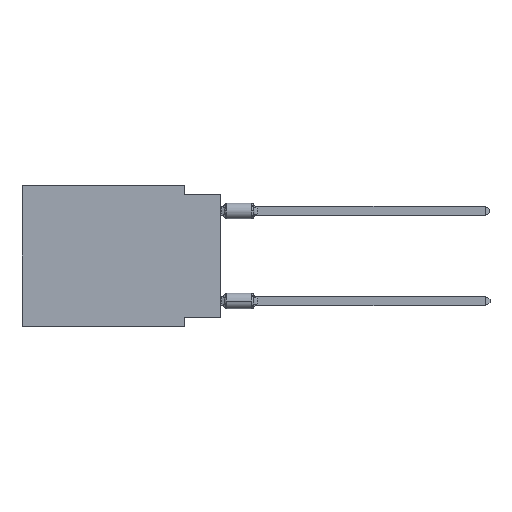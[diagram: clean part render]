
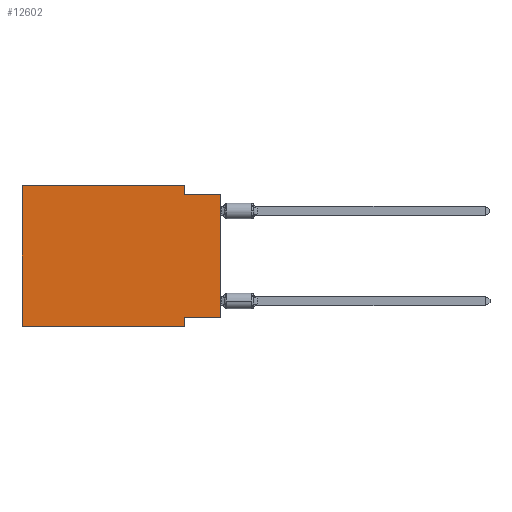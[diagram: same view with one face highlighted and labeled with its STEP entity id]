
A CAD part, left-side view. The second image highlights one B-rep face of the part: STEP entity #12602.
In plain terms, the highlighted planar face has unit normal (-1, 0, 0).
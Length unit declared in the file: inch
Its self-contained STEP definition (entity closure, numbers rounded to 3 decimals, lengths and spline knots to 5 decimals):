
#134 = EDGE_CURVE ( 'NONE', #1493, #5628, #2994, .T. ) ;
#543 = ORIENTED_EDGE ( 'NONE', *, *, #12047, .T. ) ;
#693 = VECTOR ( 'NONE', #1658, 39.37008 ) ;
#813 = CARTESIAN_POINT ( 'NONE',  ( 0., 0., -0.025 ) ) ;
#905 = DIRECTION ( 'NONE',  ( 1., 0., 0. ) ) ;
#923 = VERTEX_POINT ( 'NONE', #1410 ) ;
#1098 = AXIS2_PLACEMENT_3D ( 'NONE', #5638, #905, #8015 ) ;
#1410 = CARTESIAN_POINT ( 'NONE',  ( 0., 0.55, -0.39 ) ) ;
#1446 = LINE ( 'NONE', #2656, #15332 ) ;
#1493 = VERTEX_POINT ( 'NONE', #8475 ) ;
#1600 = DIRECTION ( 'NONE',  ( 0., 0., -1. ) ) ;
#1658 = DIRECTION ( 'NONE',  ( 0., 0., -1. ) ) ;
#2027 = PLANE ( 'NONE',  #1098 ) ;
#2193 = EDGE_CURVE ( 'NONE', #923, #12977, #14083, .T. ) ;
#2345 = CARTESIAN_POINT ( 'NONE',  ( 0., 0.1, -0.365 ) ) ;
#2633 = VERTEX_POINT ( 'NONE', #9873 ) ;
#2656 = CARTESIAN_POINT ( 'NONE',  ( 0., 0.55, -0.39 ) ) ;
#2994 = LINE ( 'NONE', #813, #4068 ) ;
#3099 = CARTESIAN_POINT ( 'NONE',  ( 0., 0.1, -0.39 ) ) ;
#3750 = VECTOR ( 'NONE', #5693, 39.37008 ) ;
#3869 = DIRECTION ( 'NONE',  ( 0., -1., 0. ) ) ;
#3892 = CARTESIAN_POINT ( 'NONE',  ( 0., 0.55, 0. ) ) ;
#4068 = VECTOR ( 'NONE', #12791, 39.37008 ) ;
#4273 = ORIENTED_EDGE ( 'NONE', *, *, #10025, .F. ) ;
#4660 = EDGE_CURVE ( 'NONE', #11105, #1493, #12467, .T. ) ;
#4673 = LINE ( 'NONE', #10883, #14875 ) ;
#4889 = VECTOR ( 'NONE', #6450, 39.37008 ) ;
#5107 = EDGE_LOOP ( 'NONE', ( #8336, #7404, #12981, #10629, #8764, #543, #8129, #4273 ) ) ;
#5628 = VERTEX_POINT ( 'NONE', #10323 ) ;
#5638 = CARTESIAN_POINT ( 'NONE',  ( 0., 0.55, 0. ) ) ;
#5693 = DIRECTION ( 'NONE',  ( 0., -1., 0. ) ) ;
#6450 = DIRECTION ( 'NONE',  ( 0., 0., 1. ) ) ;
#6956 = EDGE_CURVE ( 'NONE', #12977, #11105, #10717, .T. ) ;
#7404 = ORIENTED_EDGE ( 'NONE', *, *, #134, .F. ) ;
#7651 = CARTESIAN_POINT ( 'NONE',  ( 0., 0.55, 0. ) ) ;
#8015 = DIRECTION ( 'NONE',  ( 0., 0., -1. ) ) ;
#8122 = VECTOR ( 'NONE', #1600, 39.37008 ) ;
#8129 = ORIENTED_EDGE ( 'NONE', *, *, #8997, .F. ) ;
#8336 = ORIENTED_EDGE ( 'NONE', *, *, #10468, .T. ) ;
#8475 = CARTESIAN_POINT ( 'NONE',  ( 0., 0.1, -0.025 ) ) ;
#8764 = ORIENTED_EDGE ( 'NONE', *, *, #2193, .F. ) ;
#8997 = EDGE_CURVE ( 'NONE', #10107, #2633, #12604, .T. ) ;
#9092 = LINE ( 'NONE', #10972, #12335 ) ;
#9355 = CARTESIAN_POINT ( 'NONE',  ( 0., 0.55, 0. ) ) ;
#9766 = DIRECTION ( 'NONE',  ( 0., 1., 0. ) ) ;
#9873 = CARTESIAN_POINT ( 'NONE',  ( 0., 0.1, -0.39 ) ) ;
#10025 = EDGE_CURVE ( 'NONE', #10238, #10107, #4673, .T. ) ;
#10107 = VERTEX_POINT ( 'NONE', #2345 ) ;
#10238 = VERTEX_POINT ( 'NONE', #12919 ) ;
#10323 = CARTESIAN_POINT ( 'NONE',  ( 0., 0., -0.025 ) ) ;
#10468 = EDGE_CURVE ( 'NONE', #10238, #5628, #9092, .T. ) ;
#10629 = ORIENTED_EDGE ( 'NONE', *, *, #6956, .F. ) ;
#10717 = LINE ( 'NONE', #9355, #3750 ) ;
#10883 = CARTESIAN_POINT ( 'NONE',  ( 0., 0., -0.365 ) ) ;
#10972 = CARTESIAN_POINT ( 'NONE',  ( 0., 0., 0. ) ) ;
#11105 = VERTEX_POINT ( 'NONE', #14341 ) ;
#11422 = DIRECTION ( 'NONE',  ( 0., 0., 1. ) ) ;
#12047 = EDGE_CURVE ( 'NONE', #923, #2633, #1446, .T. ) ;
#12335 = VECTOR ( 'NONE', #11422, 39.37008 ) ;
#12467 = LINE ( 'NONE', #12684, #8122 ) ;
#12602 = ADVANCED_FACE ( 'NONE', ( #14004 ), #2027, .F. ) ;
#12604 = LINE ( 'NONE', #3099, #693 ) ;
#12684 = CARTESIAN_POINT ( 'NONE',  ( 0., 0.1, 0. ) ) ;
#12791 = DIRECTION ( 'NONE',  ( 0., -1., 0. ) ) ;
#12919 = CARTESIAN_POINT ( 'NONE',  ( 0., 0., -0.365 ) ) ;
#12977 = VERTEX_POINT ( 'NONE', #3892 ) ;
#12981 = ORIENTED_EDGE ( 'NONE', *, *, #4660, .F. ) ;
#14004 = FACE_OUTER_BOUND ( 'NONE', #5107, .T. ) ;
#14083 = LINE ( 'NONE', #7651, #4889 ) ;
#14341 = CARTESIAN_POINT ( 'NONE',  ( 0., 0.1, 0. ) ) ;
#14875 = VECTOR ( 'NONE', #9766, 39.37008 ) ;
#15332 = VECTOR ( 'NONE', #3869, 39.37008 ) ;
